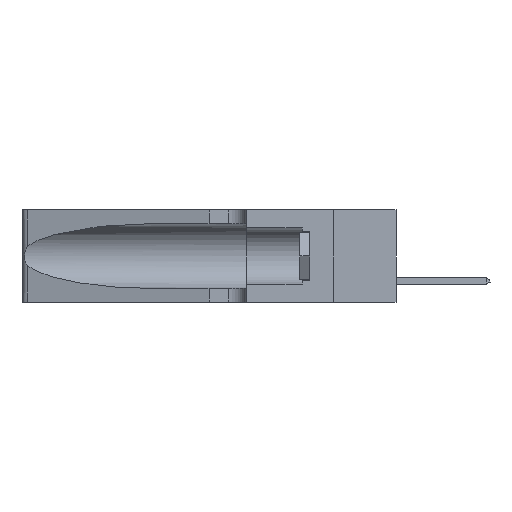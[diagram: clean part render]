
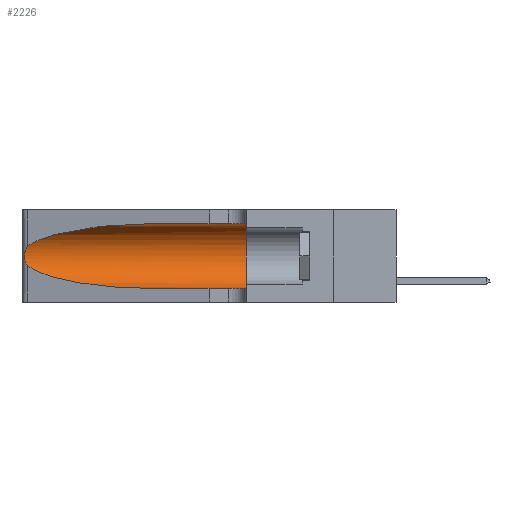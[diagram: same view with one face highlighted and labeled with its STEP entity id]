
A CAD part, left-side view. The second image highlights one B-rep face of the part: STEP entity #2226.
In plain terms, the highlighted cylindrical face has radius 3.308 mm (diameter 6.617 mm), a partial arc.
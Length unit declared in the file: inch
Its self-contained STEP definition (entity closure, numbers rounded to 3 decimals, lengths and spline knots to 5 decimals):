
#175 = LINE ( 'NONE', #11529, #12701 ) ;
#1095 = VERTEX_POINT ( 'NONE', #16938 ) ;
#1166 =( BOUNDED_CURVE ( )  B_SPLINE_CURVE ( 3, ( #34935, #12968, #34470, #10937 ),
 .UNSPECIFIED., .F., .F. ) 
 B_SPLINE_CURVE_WITH_KNOTS ( ( 4, 4 ),
 ( 1.5708, 2.84003 ),
 .UNSPECIFIED. ) 
 CURVE ( )  GEOMETRIC_REPRESENTATION_ITEM ( )  RATIONAL_B_SPLINE_CURVE ( ( 1., 0.87, 0.87, 1. ) ) 
 REPRESENTATION_ITEM ( '' )  );
#1682 = VERTEX_POINT ( 'NONE', #33489 ) ;
#2226 = ADVANCED_FACE ( 'NONE', ( #13480 ), #6954, .F. ) ;
#5931 = CARTESIAN_POINT ( 'NONE',  ( 0.25639, 1.23184, 0.21858 ) ) ;
#6213 = CARTESIAN_POINT ( 'NONE',  ( 0.26018, 1.23835, 0.19895 ) ) ;
#6742 = DIRECTION ( 'NONE',  ( 0., 1., 0. ) ) ;
#6856 = ORIENTED_EDGE ( 'NONE', *, *, #29676, .T. ) ;
#6954 = CYLINDRICAL_SURFACE ( 'NONE', #37825, 0.13025 ) ;
#6963 = EDGE_CURVE ( 'NONE', #9713, #42404, #9818, .T. ) ;
#9322 = ORIENTED_EDGE ( 'NONE', *, *, #19570, .F. ) ;
#9702 = CARTESIAN_POINT ( 'NONE',  ( 0.25639, 1.23186, 0.15144 ) ) ;
#9713 = VERTEX_POINT ( 'NONE', #16176 ) ;
#9818 =( BOUNDED_CURVE ( )  B_SPLINE_CURVE ( 3, ( #10048, #13507, #37785, #41403 ),
 .UNSPECIFIED., .F., .T. ) 
 B_SPLINE_CURVE_WITH_KNOTS ( ( 4, 4 ),
 ( 3.44316, 4.71239 ),
 .UNSPECIFIED. ) 
 CURVE ( )  GEOMETRIC_REPRESENTATION_ITEM ( )  RATIONAL_B_SPLINE_CURVE ( ( 1., 0.87, 0.87, 1. ) ) 
 REPRESENTATION_ITEM ( '' )  );
#10048 = CARTESIAN_POINT ( 'NONE',  ( 0.25487, 1.22718, 0.14631 ) ) ;
#10645 = DIRECTION ( 'NONE',  ( 0., 0., 1. ) ) ;
#10937 = CARTESIAN_POINT ( 'NONE',  ( 0.25487, 1.22718, 0.22369 ) ) ;
#11529 = CARTESIAN_POINT ( 'NONE',  ( 0.1305, 1.61858, 0.31525 ) ) ;
#12346 = VERTEX_POINT ( 'NONE', #27048 ) ;
#12701 = VECTOR ( 'NONE', #35777, 39.37008 ) ;
#12968 = CARTESIAN_POINT ( 'NONE',  ( 0.18966, 0.96281, 0.31525 ) ) ;
#13039 = CARTESIAN_POINT ( 'NONE',  ( 0.25555, 1.22994, 0.2215 ) ) ;
#13480 = FACE_OUTER_BOUND ( 'NONE', #21988, .T. ) ;
#13507 = CARTESIAN_POINT ( 'NONE',  ( 0.2373, 1.15595, 0.08982 ) ) ;
#14046 = CARTESIAN_POINT ( 'NONE',  ( 0.1305, 1.61858, 0.185 ) ) ;
#14308 = AXIS2_PLACEMENT_3D ( 'NONE', #41441, #6742, #10645 ) ;
#16036 = CARTESIAN_POINT ( 'NONE',  ( 0.25787, 1.23484, 0.2124 ) ) ;
#16176 = CARTESIAN_POINT ( 'NONE',  ( 0.25487, 1.22718, 0.14631 ) ) ;
#16494 = CARTESIAN_POINT ( 'NONE',  ( 0.26075, 1.23896, 0.19203 ) ) ;
#16643 = CARTESIAN_POINT ( 'NONE',  ( 0.25789, 1.23486, 0.15765 ) ) ;
#16938 = CARTESIAN_POINT ( 'NONE',  ( 0.1305, 0.72297, 0.31525 ) ) ;
#19497 = EDGE_CURVE ( 'NONE', #1095, #1682, #1166, .T. ) ;
#19540 = CARTESIAN_POINT ( 'NONE',  ( 0.25854, 1.2359, 0.20912 ) ) ;
#19570 = EDGE_CURVE ( 'NONE', #1095, #33076, #175, .T. ) ;
#19686 = CARTESIAN_POINT ( 'NONE',  ( 0.25555, 1.22993, 0.14849 ) ) ;
#19851 = CARTESIAN_POINT ( 'NONE',  ( 0.1305, 0.35, 0.31525 ) ) ;
#19998 = CARTESIAN_POINT ( 'NONE',  ( 0.26017, 1.23833, 0.17102 ) ) ;
#21988 = EDGE_LOOP ( 'NONE', ( #30793, #33366, #41003, #6856, #26912, #9322 ) ) ;
#24238 = DIRECTION ( 'NONE',  ( 0., 0., -1. ) ) ;
#26683 = CARTESIAN_POINT ( 'NONE',  ( 0.25487, 1.22718, 0.22369 ) ) ;
#26912 = ORIENTED_EDGE ( 'NONE', *, *, #37454, .F. ) ;
#27048 = CARTESIAN_POINT ( 'NONE',  ( 0.1305, 0.35, 0.05475 ) ) ;
#27299 = B_SPLINE_CURVE_WITH_KNOTS ( 'NONE', 3,
 ( #26683, #13039, #5931, #16036, #19540, #6213, #16494, #40796, #19998, #30460, #16643, #9702, #19686, #43965 ),
 .UNSPECIFIED., .F., .F.,
 ( 4, 2, 2, 2, 2, 2, 4 ),
 ( 0., 0.00027, 0.00053, 0.00107, 0.0016, 0.00187, 0.00214 ),
 .UNSPECIFIED. ) ;
#29676 = EDGE_CURVE ( 'NONE', #42404, #12346, #30228, .T. ) ;
#29701 = VECTOR ( 'NONE', #41854, 39.37008 ) ;
#29946 = EDGE_CURVE ( 'NONE', #1682, #9713, #27299, .T. ) ;
#30228 = LINE ( 'NONE', #41423, #29701 ) ;
#30460 = CARTESIAN_POINT ( 'NONE',  ( 0.25856, 1.23593, 0.16098 ) ) ;
#30793 = ORIENTED_EDGE ( 'NONE', *, *, #19497, .T. ) ;
#31515 = DIRECTION ( 'NONE',  ( 0., -1., 0. ) ) ;
#33076 = VERTEX_POINT ( 'NONE', #19851 ) ;
#33366 = ORIENTED_EDGE ( 'NONE', *, *, #29946, .T. ) ;
#33489 = CARTESIAN_POINT ( 'NONE',  ( 0.25487, 1.22718, 0.22369 ) ) ;
#34470 = CARTESIAN_POINT ( 'NONE',  ( 0.2373, 1.15595, 0.28018 ) ) ;
#34542 = CARTESIAN_POINT ( 'NONE',  ( 0.1305, 0.72297, 0.05475 ) ) ;
#34935 = CARTESIAN_POINT ( 'NONE',  ( 0.1305, 0.72297, 0.31525 ) ) ;
#35777 = DIRECTION ( 'NONE',  ( 0., -1., 0. ) ) ;
#37454 = EDGE_CURVE ( 'NONE', #33076, #12346, #39498, .T. ) ;
#37785 = CARTESIAN_POINT ( 'NONE',  ( 0.18966, 0.96281, 0.05475 ) ) ;
#37825 = AXIS2_PLACEMENT_3D ( 'NONE', #14046, #31515, #24238 ) ;
#39498 = CIRCLE ( 'NONE', #14308, 0.13025 ) ;
#40796 = CARTESIAN_POINT ( 'NONE',  ( 0.26075, 1.23896, 0.178 ) ) ;
#41003 = ORIENTED_EDGE ( 'NONE', *, *, #6963, .T. ) ;
#41403 = CARTESIAN_POINT ( 'NONE',  ( 0.1305, 0.72297, 0.05475 ) ) ;
#41423 = CARTESIAN_POINT ( 'NONE',  ( 0.1305, 1.61858, 0.05475 ) ) ;
#41441 = CARTESIAN_POINT ( 'NONE',  ( 0.1305, 0.35, 0.185 ) ) ;
#41854 = DIRECTION ( 'NONE',  ( 0., -1., 0. ) ) ;
#42404 = VERTEX_POINT ( 'NONE', #34542 ) ;
#43965 = CARTESIAN_POINT ( 'NONE',  ( 0.25487, 1.22718, 0.14631 ) ) ;
